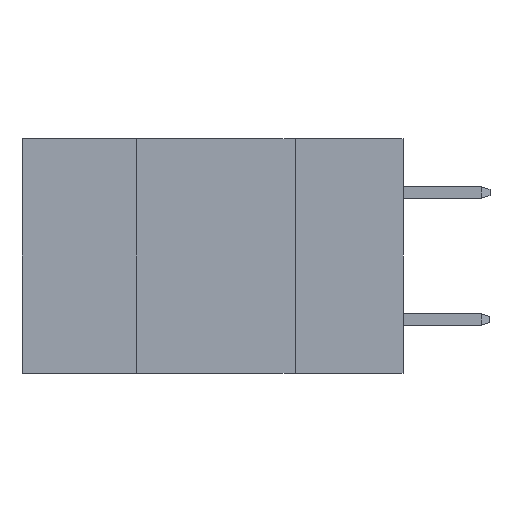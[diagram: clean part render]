
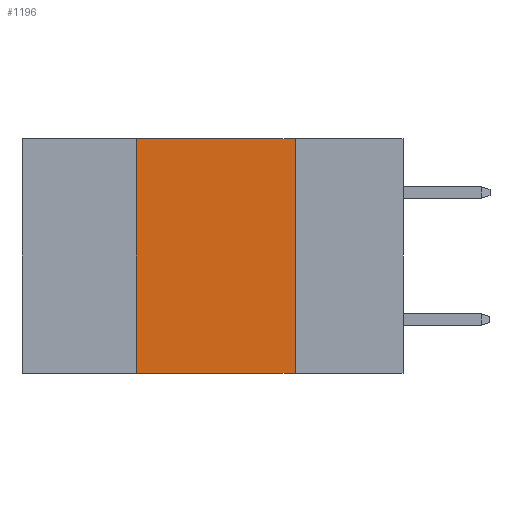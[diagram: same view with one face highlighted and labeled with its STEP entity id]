
A CAD part, left-side view. The second image highlights one B-rep face of the part: STEP entity #1196.
In plain terms, the highlighted planar face has unit normal (-1, 0, 0).
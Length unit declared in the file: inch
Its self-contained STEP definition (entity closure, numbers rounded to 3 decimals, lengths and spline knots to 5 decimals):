
#105 = VERTEX_POINT ( 'NONE', #5863 ) ;
#159 = CARTESIAN_POINT ( 'NONE',  ( 0., 0.42, -0.37 ) ) ;
#392 = VECTOR ( 'NONE', #6394, 39.37008 ) ;
#600 = CARTESIAN_POINT ( 'NONE',  ( 0., 0.17, 0. ) ) ;
#717 = CARTESIAN_POINT ( 'NONE',  ( 0., 0.6, -0.37 ) ) ;
#1196 = ADVANCED_FACE ( 'NONE', ( #7309 ), #6643, .F. ) ;
#1575 = EDGE_CURVE ( 'NONE', #6760, #4520, #9692, .T. ) ;
#2006 = AXIS2_PLACEMENT_3D ( 'NONE', #5755, #3050, #10857 ) ;
#2021 = CARTESIAN_POINT ( 'NONE',  ( 0., 0.42, 0. ) ) ;
#2116 = VERTEX_POINT ( 'NONE', #10879 ) ;
#2271 = ORIENTED_EDGE ( 'NONE', *, *, #6034, .F. ) ;
#3050 = DIRECTION ( 'NONE',  ( 1., 0., 0. ) ) ;
#3267 = ORIENTED_EDGE ( 'NONE', *, *, #7044, .T. ) ;
#4063 = DIRECTION ( 'NONE',  ( 0., 0., -1. ) ) ;
#4426 = EDGE_CURVE ( 'NONE', #2116, #105, #9134, .T. ) ;
#4520 = VERTEX_POINT ( 'NONE', #8471 ) ;
#4555 = LINE ( 'NONE', #9684, #392 ) ;
#4851 = DIRECTION ( 'NONE',  ( 0., -1., 0. ) ) ;
#5474 = DIRECTION ( 'NONE',  ( 0., 0., 1. ) ) ;
#5755 = CARTESIAN_POINT ( 'NONE',  ( 0., 0.6, 0. ) ) ;
#5863 = CARTESIAN_POINT ( 'NONE',  ( 0., 0.17, -0.37 ) ) ;
#6034 = EDGE_CURVE ( 'NONE', #4520, #2116, #4555, .T. ) ;
#6394 = DIRECTION ( 'NONE',  ( 0., -1., 0. ) ) ;
#6425 = ORIENTED_EDGE ( 'NONE', *, *, #4426, .F. ) ;
#6601 = VECTOR ( 'NONE', #4851, 39.37008 ) ;
#6643 = PLANE ( 'NONE',  #2006 ) ;
#6760 = VERTEX_POINT ( 'NONE', #159 ) ;
#6886 = ORIENTED_EDGE ( 'NONE', *, *, #1575, .F. ) ;
#7044 = EDGE_CURVE ( 'NONE', #6760, #105, #8357, .T. ) ;
#7309 = FACE_OUTER_BOUND ( 'NONE', #7354, .T. ) ;
#7354 = EDGE_LOOP ( 'NONE', ( #6425, #2271, #6886, #3267 ) ) ;
#7572 = VECTOR ( 'NONE', #5474, 39.37008 ) ;
#8357 = LINE ( 'NONE', #717, #6601 ) ;
#8471 = CARTESIAN_POINT ( 'NONE',  ( 0., 0.42, 0. ) ) ;
#9134 = LINE ( 'NONE', #600, #9875 ) ;
#9684 = CARTESIAN_POINT ( 'NONE',  ( 0., 0.6, 0. ) ) ;
#9692 = LINE ( 'NONE', #2021, #7572 ) ;
#9875 = VECTOR ( 'NONE', #4063, 39.37008 ) ;
#10857 = DIRECTION ( 'NONE',  ( 0., 0., -1. ) ) ;
#10879 = CARTESIAN_POINT ( 'NONE',  ( 0., 0.17, 0. ) ) ;
